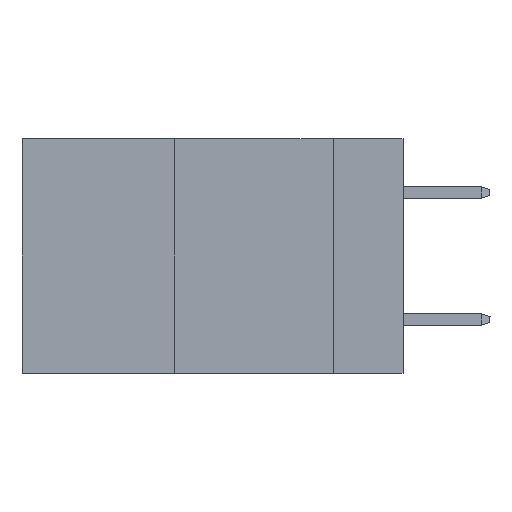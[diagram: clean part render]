
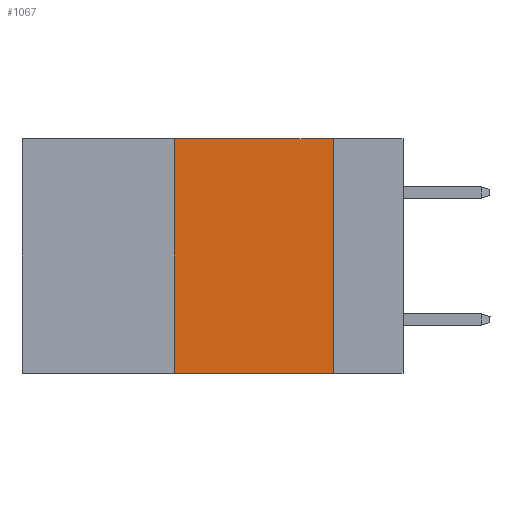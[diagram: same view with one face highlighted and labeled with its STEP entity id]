
A CAD part, left-side view. The second image highlights one B-rep face of the part: STEP entity #1067.
In plain terms, the highlighted planar face has unit normal (-1, 0, 0).
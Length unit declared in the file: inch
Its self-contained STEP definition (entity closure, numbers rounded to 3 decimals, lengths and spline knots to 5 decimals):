
#3 = CARTESIAN_POINT ( 'NONE',  ( 0., 0.11, -0.37 ) ) ;
#701 = CARTESIAN_POINT ( 'NONE',  ( 0., 0.36, 0. ) ) ;
#1067 = ADVANCED_FACE ( 'NONE', ( #14201 ), #2513, .F. ) ;
#1180 = DIRECTION ( 'NONE',  ( 0., 0., -1. ) ) ;
#1789 = AXIS2_PLACEMENT_3D ( 'NONE', #11920, #3468, #1180 ) ;
#2513 = PLANE ( 'NONE',  #1789 ) ;
#2951 = LINE ( 'NONE', #13906, #8817 ) ;
#3107 = DIRECTION ( 'NONE',  ( 0., -1., 0. ) ) ;
#3468 = DIRECTION ( 'NONE',  ( 1., 0., 0. ) ) ;
#3552 = DIRECTION ( 'NONE',  ( 0., -1., 0. ) ) ;
#3850 = EDGE_LOOP ( 'NONE', ( #11847, #9335, #14748, #10959 ) ) ;
#5577 = VERTEX_POINT ( 'NONE', #5765 ) ;
#5601 = LINE ( 'NONE', #9069, #6917 ) ;
#5765 = CARTESIAN_POINT ( 'NONE',  ( 0., 0.11, 0. ) ) ;
#5835 = EDGE_CURVE ( 'NONE', #9200, #6441, #2951, .T. ) ;
#6111 = LINE ( 'NONE', #9503, #9230 ) ;
#6441 = VERTEX_POINT ( 'NONE', #3 ) ;
#6917 = VECTOR ( 'NONE', #14957, 39.37008 ) ;
#8255 = CARTESIAN_POINT ( 'NONE',  ( 0., 0.6, 0. ) ) ;
#8770 = EDGE_CURVE ( 'NONE', #11043, #5577, #9515, .T. ) ;
#8817 = VECTOR ( 'NONE', #3107, 39.37008 ) ;
#9069 = CARTESIAN_POINT ( 'NONE',  ( 0., 0.11, 0. ) ) ;
#9200 = VERTEX_POINT ( 'NONE', #12793 ) ;
#9230 = VECTOR ( 'NONE', #10886, 39.37008 ) ;
#9335 = ORIENTED_EDGE ( 'NONE', *, *, #8770, .F. ) ;
#9503 = CARTESIAN_POINT ( 'NONE',  ( 0., 0.36, 0. ) ) ;
#9515 = LINE ( 'NONE', #8255, #10629 ) ;
#10629 = VECTOR ( 'NONE', #3552, 39.37008 ) ;
#10886 = DIRECTION ( 'NONE',  ( 0., 0., 1. ) ) ;
#10959 = ORIENTED_EDGE ( 'NONE', *, *, #5835, .T. ) ;
#11043 = VERTEX_POINT ( 'NONE', #701 ) ;
#11847 = ORIENTED_EDGE ( 'NONE', *, *, #12031, .F. ) ;
#11920 = CARTESIAN_POINT ( 'NONE',  ( 0., 0.6, 0. ) ) ;
#12031 = EDGE_CURVE ( 'NONE', #5577, #6441, #5601, .T. ) ;
#12793 = CARTESIAN_POINT ( 'NONE',  ( 0., 0.36, -0.37 ) ) ;
#13906 = CARTESIAN_POINT ( 'NONE',  ( 0., 0.6, -0.37 ) ) ;
#14201 = FACE_OUTER_BOUND ( 'NONE', #3850, .T. ) ;
#14236 = EDGE_CURVE ( 'NONE', #9200, #11043, #6111, .T. ) ;
#14748 = ORIENTED_EDGE ( 'NONE', *, *, #14236, .F. ) ;
#14957 = DIRECTION ( 'NONE',  ( 0., 0., -1. ) ) ;
